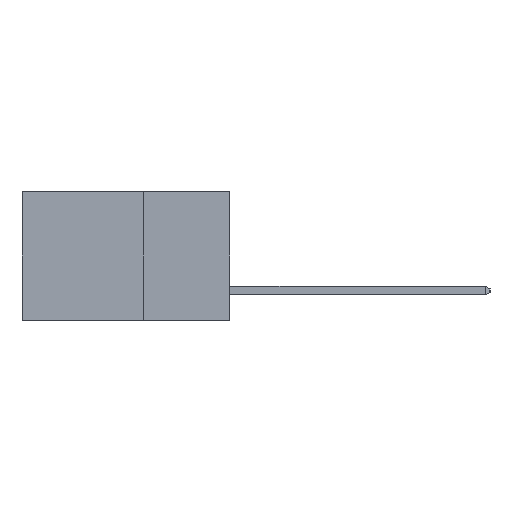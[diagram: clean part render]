
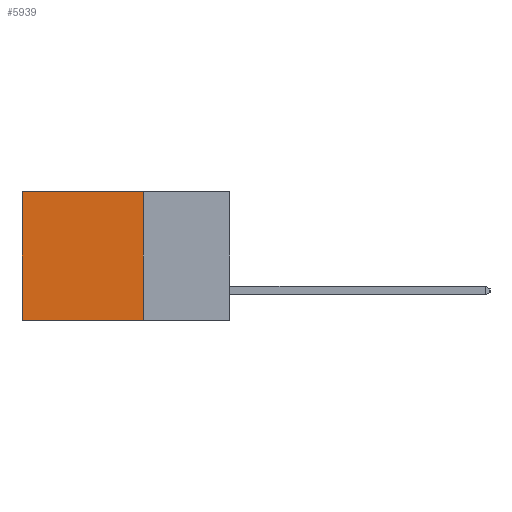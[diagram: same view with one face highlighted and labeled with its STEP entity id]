
A CAD part, left-side view. The second image highlights one B-rep face of the part: STEP entity #5939.
In plain terms, the highlighted planar face has unit normal (-1, 0, 0).
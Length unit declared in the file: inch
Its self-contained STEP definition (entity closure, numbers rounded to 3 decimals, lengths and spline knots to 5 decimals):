
#573 = CARTESIAN_POINT ( 'NONE',  ( 0.298, 0.6, 0. ) ) ;
#579 = DIRECTION ( 'NONE',  ( 0., 1., 0. ) ) ;
#1052 = ORIENTED_EDGE ( 'NONE', *, *, #3299, .T. ) ;
#1083 = CARTESIAN_POINT ( 'NONE',  ( 0.298, 0.25, -0.37 ) ) ;
#1426 = VECTOR ( 'NONE', #8199, 39.37008 ) ;
#2348 = EDGE_CURVE ( 'NONE', #14376, #11849, #10132, .T. ) ;
#2661 = VECTOR ( 'NONE', #7911, 39.37008 ) ;
#3299 = EDGE_CURVE ( 'NONE', #4726, #11849, #11468, .T. ) ;
#3377 = AXIS2_PLACEMENT_3D ( 'NONE', #14703, #15948, #8492 ) ;
#3669 = FACE_OUTER_BOUND ( 'NONE', #6875, .T. ) ;
#4061 = DIRECTION ( 'NONE',  ( 0., 0., -1. ) ) ;
#4567 = CARTESIAN_POINT ( 'NONE',  ( 0.298, 0.6, 0. ) ) ;
#4726 = VERTEX_POINT ( 'NONE', #4567 ) ;
#5270 = CARTESIAN_POINT ( 'NONE',  ( 0.298, 0.25, 0. ) ) ;
#5741 = ORIENTED_EDGE ( 'NONE', *, *, #11025, .T. ) ;
#5856 = VECTOR ( 'NONE', #4061, 39.37008 ) ;
#5939 = ADVANCED_FACE ( 'NONE', ( #3669 ), #7225, .F. ) ;
#6875 = EDGE_LOOP ( 'NONE', ( #1052, #8297, #12441, #5741 ) ) ;
#6876 = VECTOR ( 'NONE', #579, 39.37008 ) ;
#7225 = PLANE ( 'NONE',  #3377 ) ;
#7311 = CARTESIAN_POINT ( 'NONE',  ( 0.298, 0.25, 0. ) ) ;
#7911 = DIRECTION ( 'NONE',  ( 0., 1., 0. ) ) ;
#8199 = DIRECTION ( 'NONE',  ( 0., 0., -1. ) ) ;
#8297 = ORIENTED_EDGE ( 'NONE', *, *, #2348, .F. ) ;
#8492 = DIRECTION ( 'NONE',  ( 0., 0., -1. ) ) ;
#9218 = CARTESIAN_POINT ( 'NONE',  ( 0.298, 0.25, -0.37 ) ) ;
#10132 = LINE ( 'NONE', #1083, #2661 ) ;
#10204 = LINE ( 'NONE', #11889, #6876 ) ;
#11025 = EDGE_CURVE ( 'NONE', #15330, #4726, #10204, .T. ) ;
#11468 = LINE ( 'NONE', #573, #1426 ) ;
#11849 = VERTEX_POINT ( 'NONE', #14216 ) ;
#11889 = CARTESIAN_POINT ( 'NONE',  ( 0.298, 0.25, 0. ) ) ;
#12441 = ORIENTED_EDGE ( 'NONE', *, *, #14296, .F. ) ;
#12542 = LINE ( 'NONE', #5270, #5856 ) ;
#14216 = CARTESIAN_POINT ( 'NONE',  ( 0.298, 0.6, -0.37 ) ) ;
#14296 = EDGE_CURVE ( 'NONE', #15330, #14376, #12542, .T. ) ;
#14376 = VERTEX_POINT ( 'NONE', #9218 ) ;
#14703 = CARTESIAN_POINT ( 'NONE',  ( 0.298, 0.25, 0. ) ) ;
#15330 = VERTEX_POINT ( 'NONE', #7311 ) ;
#15948 = DIRECTION ( 'NONE',  ( 1., 0., 0. ) ) ;
